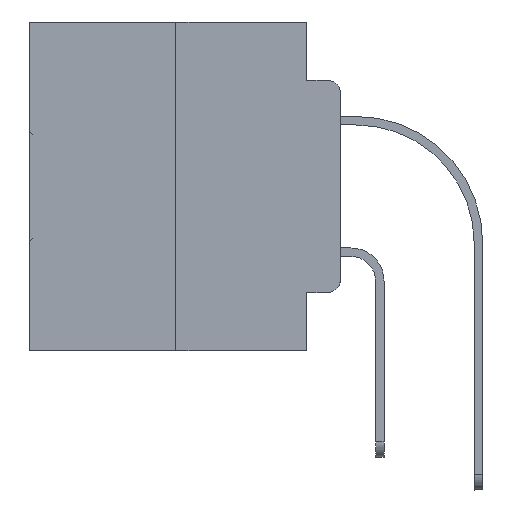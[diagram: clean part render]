
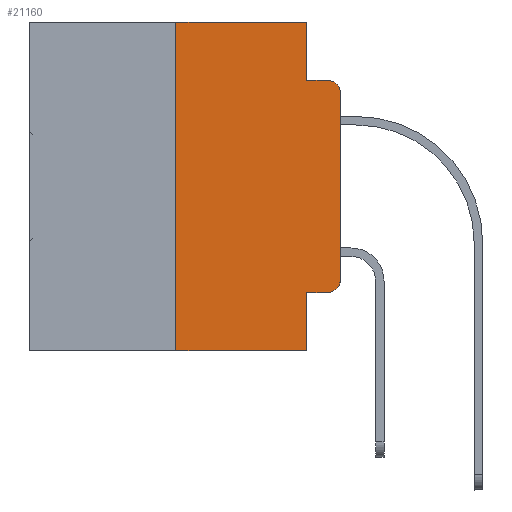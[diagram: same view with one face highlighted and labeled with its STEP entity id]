
A CAD part, left-side view. The second image highlights one B-rep face of the part: STEP entity #21160.
In plain terms, the highlighted planar face has unit normal (-1, 0, 0).
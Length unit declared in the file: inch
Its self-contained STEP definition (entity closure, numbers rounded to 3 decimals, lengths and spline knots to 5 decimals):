
#204 = EDGE_CURVE ( 'NONE', #13720, #17448, #9714, .T. ) ;
#297 = PLANE ( 'NONE',  #29149 ) ;
#691 = CARTESIAN_POINT ( 'NONE',  ( 0., 0.25, -0.5 ) ) ;
#1173 = DIRECTION ( 'NONE',  ( 0., -1., 0. ) ) ;
#1272 = EDGE_CURVE ( 'NONE', #23934, #3169, #18003, .T. ) ;
#1318 = VERTEX_POINT ( 'NONE', #24323 ) ;
#1495 = LINE ( 'NONE', #6380, #25198 ) ;
#1551 = LINE ( 'NONE', #32531, #24136 ) ;
#2108 = DIRECTION ( 'NONE',  ( 0., -1., 0. ) ) ;
#2253 = CARTESIAN_POINT ( 'NONE',  ( 0., 0.051, 0. ) ) ;
#2626 = EDGE_CURVE ( 'NONE', #22485, #3169, #24836, .T. ) ;
#2680 = VERTEX_POINT ( 'NONE', #14786 ) ;
#3169 = VERTEX_POINT ( 'NONE', #15567 ) ;
#3535 = EDGE_CURVE ( 'NONE', #2680, #16156, #22237, .T. ) ;
#3600 = CARTESIAN_POINT ( 'NONE',  ( 0., 0.02, -0.4115 ) ) ;
#4545 = EDGE_LOOP ( 'NONE', ( #32470, #23699, #32852, #21161, #27892, #18428, #27195, #14841, #8495, #6633 ) ) ;
#4706 = DIRECTION ( 'NONE',  ( 0., -1., 0. ) ) ;
#4748 = VECTOR ( 'NONE', #30287, 39.37008 ) ;
#4861 = FACE_OUTER_BOUND ( 'NONE', #4545, .T. ) ;
#5406 = CARTESIAN_POINT ( 'NONE',  ( 0., 0.02, -0.1085 ) ) ;
#5829 = CIRCLE ( 'NONE', #14419, 0.02 ) ;
#6380 = CARTESIAN_POINT ( 'NONE',  ( 0., 0.473, 0. ) ) ;
#6633 = ORIENTED_EDGE ( 'NONE', *, *, #24605, .T. ) ;
#7135 = DIRECTION ( 'NONE',  ( 0., 0., -1. ) ) ;
#7860 = EDGE_CURVE ( 'NONE', #17448, #30086, #1495, .T. ) ;
#7954 = EDGE_CURVE ( 'NONE', #13720, #14736, #13606, .T. ) ;
#8065 = VECTOR ( 'NONE', #4706, 39.37008 ) ;
#8495 = ORIENTED_EDGE ( 'NONE', *, *, #3535, .T. ) ;
#8836 = VECTOR ( 'NONE', #11251, 39.37008 ) ;
#9154 = LINE ( 'NONE', #22222, #15323 ) ;
#9714 = LINE ( 'NONE', #19933, #4748 ) ;
#10287 = EDGE_CURVE ( 'NONE', #30086, #22485, #9154, .T. ) ;
#11251 = DIRECTION ( 'NONE',  ( 0., -1., 0. ) ) ;
#12783 = VECTOR ( 'NONE', #13625, 39.37008 ) ;
#13606 = LINE ( 'NONE', #26977, #8836 ) ;
#13625 = DIRECTION ( 'NONE',  ( 0., 0., 1. ) ) ;
#13715 = EDGE_CURVE ( 'NONE', #1318, #23934, #23193, .T. ) ;
#13720 = VERTEX_POINT ( 'NONE', #691 ) ;
#14419 = AXIS2_PLACEMENT_3D ( 'NONE', #30019, #32844, #27688 ) ;
#14736 = VERTEX_POINT ( 'NONE', #16677 ) ;
#14786 = CARTESIAN_POINT ( 'NONE',  ( 0., 0.051, -0.4115 ) ) ;
#14841 = ORIENTED_EDGE ( 'NONE', *, *, #27631, .F. ) ;
#14872 = CARTESIAN_POINT ( 'NONE',  ( 0., 0.051, -0.4115 ) ) ;
#15106 = CARTESIAN_POINT ( 'NONE',  ( 0., 0.473, 0. ) ) ;
#15323 = VECTOR ( 'NONE', #7135, 39.37008 ) ;
#15483 = DIRECTION ( 'NONE',  ( -1., 0., 0. ) ) ;
#15567 = CARTESIAN_POINT ( 'NONE',  ( 0., 0.02, -0.0885 ) ) ;
#15592 = DIRECTION ( 'NONE',  ( 1., 0., 0. ) ) ;
#16156 = VERTEX_POINT ( 'NONE', #3600 ) ;
#16677 = CARTESIAN_POINT ( 'NONE',  ( 0., 0.051, -0.5 ) ) ;
#17434 = CARTESIAN_POINT ( 'NONE',  ( 0., 0., -0.1085 ) ) ;
#17448 = VERTEX_POINT ( 'NONE', #28926 ) ;
#18003 = CIRCLE ( 'NONE', #22831, 0.02 ) ;
#18275 = DIRECTION ( 'NONE',  ( 0., 0., -1. ) ) ;
#18428 = ORIENTED_EDGE ( 'NONE', *, *, #204, .F. ) ;
#19933 = CARTESIAN_POINT ( 'NONE',  ( 0., 0.25, 0. ) ) ;
#21160 = ADVANCED_FACE ( 'NONE', ( #4861 ), #297, .F. ) ;
#21161 = ORIENTED_EDGE ( 'NONE', *, *, #10287, .F. ) ;
#22033 = DIRECTION ( 'NONE',  ( 0., 0., -1. ) ) ;
#22222 = CARTESIAN_POINT ( 'NONE',  ( 0., 0.051, 0. ) ) ;
#22237 = LINE ( 'NONE', #14872, #27367 ) ;
#22485 = VERTEX_POINT ( 'NONE', #24986 ) ;
#22831 = AXIS2_PLACEMENT_3D ( 'NONE', #5406, #15483, #25697 ) ;
#23193 = LINE ( 'NONE', #23516, #12783 ) ;
#23516 = CARTESIAN_POINT ( 'NONE',  ( 0., 0., 0. ) ) ;
#23699 = ORIENTED_EDGE ( 'NONE', *, *, #1272, .T. ) ;
#23934 = VERTEX_POINT ( 'NONE', #17434 ) ;
#24136 = VECTOR ( 'NONE', #22033, 39.37008 ) ;
#24323 = CARTESIAN_POINT ( 'NONE',  ( 0., 0., -0.3915 ) ) ;
#24605 = EDGE_CURVE ( 'NONE', #16156, #1318, #5829, .T. ) ;
#24836 = LINE ( 'NONE', #32831, #8065 ) ;
#24986 = CARTESIAN_POINT ( 'NONE',  ( 0., 0.051, -0.0885 ) ) ;
#25198 = VECTOR ( 'NONE', #1173, 39.37008 ) ;
#25697 = DIRECTION ( 'NONE',  ( 0., 0., -1. ) ) ;
#26977 = CARTESIAN_POINT ( 'NONE',  ( 0., 0.473, -0.5 ) ) ;
#27195 = ORIENTED_EDGE ( 'NONE', *, *, #7954, .T. ) ;
#27367 = VECTOR ( 'NONE', #2108, 39.37008 ) ;
#27631 = EDGE_CURVE ( 'NONE', #2680, #14736, #1551, .T. ) ;
#27688 = DIRECTION ( 'NONE',  ( 0., 0., -1. ) ) ;
#27892 = ORIENTED_EDGE ( 'NONE', *, *, #7860, .F. ) ;
#28926 = CARTESIAN_POINT ( 'NONE',  ( 0., 0.25, 0. ) ) ;
#29149 = AXIS2_PLACEMENT_3D ( 'NONE', #15106, #15592, #18275 ) ;
#30019 = CARTESIAN_POINT ( 'NONE',  ( 0., 0.02, -0.3915 ) ) ;
#30086 = VERTEX_POINT ( 'NONE', #2253 ) ;
#30287 = DIRECTION ( 'NONE',  ( 0., 0., 1. ) ) ;
#32470 = ORIENTED_EDGE ( 'NONE', *, *, #13715, .T. ) ;
#32531 = CARTESIAN_POINT ( 'NONE',  ( 0., 0.051, 0. ) ) ;
#32831 = CARTESIAN_POINT ( 'NONE',  ( 0., 0.051, -0.0885 ) ) ;
#32844 = DIRECTION ( 'NONE',  ( -1., 0., 0. ) ) ;
#32852 = ORIENTED_EDGE ( 'NONE', *, *, #2626, .F. ) ;
